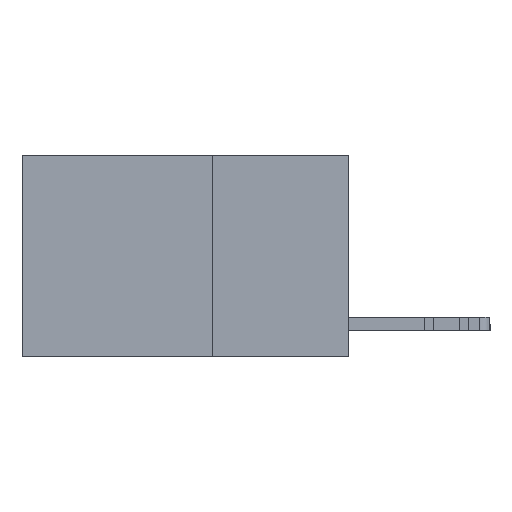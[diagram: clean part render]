
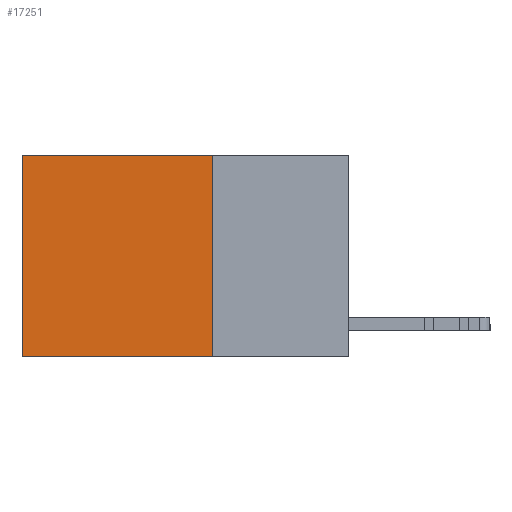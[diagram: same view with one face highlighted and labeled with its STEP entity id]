
A CAD part, left-side view. The second image highlights one B-rep face of the part: STEP entity #17251.
In plain terms, the highlighted planar face has unit normal (-1, 0, 0).
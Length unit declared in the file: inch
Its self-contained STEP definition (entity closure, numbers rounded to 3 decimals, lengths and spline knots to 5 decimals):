
#67 = VECTOR ( 'NONE', #23080, 39.37008 ) ;
#1570 = DIRECTION ( 'NONE',  ( 1., 0., 0. ) ) ;
#2160 = VECTOR ( 'NONE', #24211, 39.37008 ) ;
#4167 = LINE ( 'NONE', #16984, #27985 ) ;
#5616 = VERTEX_POINT ( 'NONE', #6024 ) ;
#6024 = CARTESIAN_POINT ( 'NONE',  ( 0.2625, 0.6, 0. ) ) ;
#7316 = CARTESIAN_POINT ( 'NONE',  ( 0.2625, 0.6, 0. ) ) ;
#7476 = EDGE_CURVE ( 'NONE', #24452, #5616, #15597, .T. ) ;
#7519 = CARTESIAN_POINT ( 'NONE',  ( 0.2625, 0.6, -0.37 ) ) ;
#8104 = VERTEX_POINT ( 'NONE', #7519 ) ;
#8499 = ORIENTED_EDGE ( 'NONE', *, *, #13114, .T. ) ;
#9088 = ORIENTED_EDGE ( 'NONE', *, *, #9843, .F. ) ;
#9843 = EDGE_CURVE ( 'NONE', #24452, #20520, #4167, .T. ) ;
#10359 = DIRECTION ( 'NONE',  ( 0., 0., -1. ) ) ;
#11963 = EDGE_CURVE ( 'NONE', #20520, #8104, #12596, .T. ) ;
#12596 = LINE ( 'NONE', #21371, #67 ) ;
#12806 = VECTOR ( 'NONE', #16096, 39.37008 ) ;
#13114 = EDGE_CURVE ( 'NONE', #5616, #8104, #27003, .T. ) ;
#14386 = PLANE ( 'NONE',  #16042 ) ;
#14506 = ORIENTED_EDGE ( 'NONE', *, *, #7476, .T. ) ;
#14818 = DIRECTION ( 'NONE',  ( 0., 0., -1. ) ) ;
#15116 = CARTESIAN_POINT ( 'NONE',  ( 0.2625, 0.25, 0. ) ) ;
#15597 = LINE ( 'NONE', #17630, #2160 ) ;
#15721 = CARTESIAN_POINT ( 'NONE',  ( 0.2625, 0.25, -0.37 ) ) ;
#16042 = AXIS2_PLACEMENT_3D ( 'NONE', #23289, #1570, #10359 ) ;
#16096 = DIRECTION ( 'NONE',  ( 0., 0., -1. ) ) ;
#16984 = CARTESIAN_POINT ( 'NONE',  ( 0.2625, 0.25, 0. ) ) ;
#17251 = ADVANCED_FACE ( 'NONE', ( #23583 ), #14386, .F. ) ;
#17630 = CARTESIAN_POINT ( 'NONE',  ( 0.2625, 0.25, 0. ) ) ;
#20520 = VERTEX_POINT ( 'NONE', #15721 ) ;
#21371 = CARTESIAN_POINT ( 'NONE',  ( 0.2625, 0.25, -0.37 ) ) ;
#22244 = EDGE_LOOP ( 'NONE', ( #8499, #23269, #9088, #14506 ) ) ;
#23080 = DIRECTION ( 'NONE',  ( 0., 1., 0. ) ) ;
#23269 = ORIENTED_EDGE ( 'NONE', *, *, #11963, .F. ) ;
#23289 = CARTESIAN_POINT ( 'NONE',  ( 0.2625, 0.25, 0. ) ) ;
#23583 = FACE_OUTER_BOUND ( 'NONE', #22244, .T. ) ;
#24211 = DIRECTION ( 'NONE',  ( 0., 1., 0. ) ) ;
#24452 = VERTEX_POINT ( 'NONE', #15116 ) ;
#27003 = LINE ( 'NONE', #7316, #12806 ) ;
#27985 = VECTOR ( 'NONE', #14818, 39.37008 ) ;
